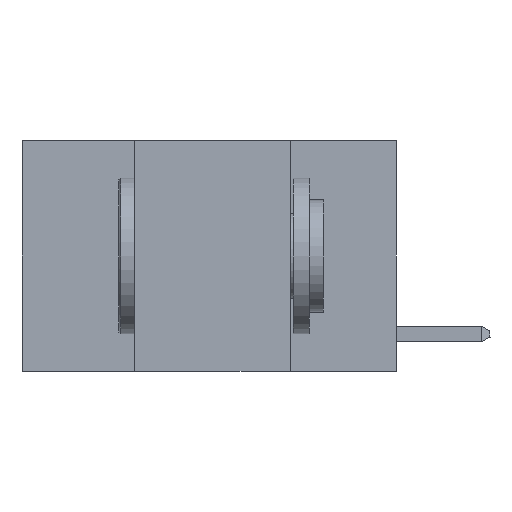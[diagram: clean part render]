
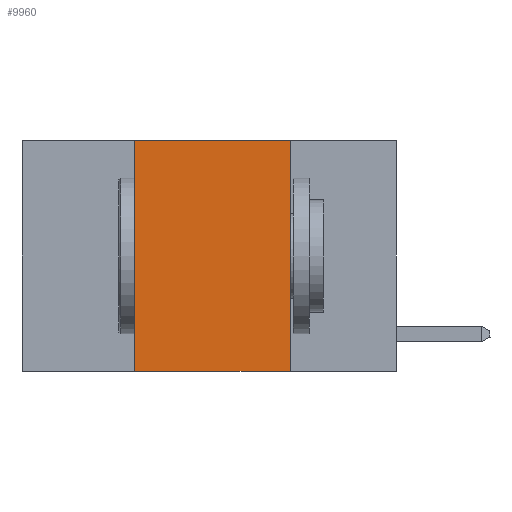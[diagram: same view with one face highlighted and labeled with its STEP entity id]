
A CAD part, left-side view. The second image highlights one B-rep face of the part: STEP entity #9960.
In plain terms, the highlighted planar face has unit normal (-1, 0, 0).
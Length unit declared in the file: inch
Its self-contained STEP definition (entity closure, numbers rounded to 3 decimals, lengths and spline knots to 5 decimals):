
#181 = DIRECTION ( 'NONE',  ( 0., 0., -1. ) ) ;
#400 = ORIENTED_EDGE ( 'NONE', *, *, #8873, .F. ) ;
#420 = LINE ( 'NONE', #10847, #8089 ) ;
#532 = DIRECTION ( 'NONE',  ( 0., -1., 0. ) ) ;
#733 = ORIENTED_EDGE ( 'NONE', *, *, #2205, .F. ) ;
#855 = LINE ( 'NONE', #8865, #3479 ) ;
#1025 = LINE ( 'NONE', #4388, #5730 ) ;
#1052 = DIRECTION ( 'NONE',  ( 1., 0., 0. ) ) ;
#1466 = ORIENTED_EDGE ( 'NONE', *, *, #10850, .F. ) ;
#2003 = VERTEX_POINT ( 'NONE', #9955 ) ;
#2205 = EDGE_CURVE ( 'NONE', #6620, #8295, #2412, .T. ) ;
#2412 = LINE ( 'NONE', #8538, #4542 ) ;
#3479 = VECTOR ( 'NONE', #5262, 39.37008 ) ;
#3792 = FACE_OUTER_BOUND ( 'NONE', #8815, .T. ) ;
#4388 = CARTESIAN_POINT ( 'NONE',  ( 0., 0.17, 0. ) ) ;
#4542 = VECTOR ( 'NONE', #532, 39.37008 ) ;
#5262 = DIRECTION ( 'NONE',  ( 0., -1., 0. ) ) ;
#5730 = VECTOR ( 'NONE', #7804, 39.37008 ) ;
#6620 = VERTEX_POINT ( 'NONE', #9179 ) ;
#7317 = ORIENTED_EDGE ( 'NONE', *, *, #7428, .T. ) ;
#7428 = EDGE_CURVE ( 'NONE', #2003, #10250, #855, .T. ) ;
#7804 = DIRECTION ( 'NONE',  ( 0., 0., -1. ) ) ;
#8089 = VECTOR ( 'NONE', #10003, 39.37008 ) ;
#8295 = VERTEX_POINT ( 'NONE', #10362 ) ;
#8538 = CARTESIAN_POINT ( 'NONE',  ( 0., 0.6, 0. ) ) ;
#8815 = EDGE_LOOP ( 'NONE', ( #400, #733, #1466, #7317 ) ) ;
#8865 = CARTESIAN_POINT ( 'NONE',  ( 0., 0.6, -0.37 ) ) ;
#8873 = EDGE_CURVE ( 'NONE', #8295, #10250, #1025, .T. ) ;
#9179 = CARTESIAN_POINT ( 'NONE',  ( 0., 0.42, 0. ) ) ;
#9765 = CARTESIAN_POINT ( 'NONE',  ( 0., 0.6, 0. ) ) ;
#9823 = PLANE ( 'NONE',  #10103 ) ;
#9851 = CARTESIAN_POINT ( 'NONE',  ( 0., 0.17, -0.37 ) ) ;
#9955 = CARTESIAN_POINT ( 'NONE',  ( 0., 0.42, -0.37 ) ) ;
#9960 = ADVANCED_FACE ( 'NONE', ( #3792 ), #9823, .F. ) ;
#10003 = DIRECTION ( 'NONE',  ( 0., 0., 1. ) ) ;
#10103 = AXIS2_PLACEMENT_3D ( 'NONE', #9765, #1052, #181 ) ;
#10250 = VERTEX_POINT ( 'NONE', #9851 ) ;
#10362 = CARTESIAN_POINT ( 'NONE',  ( 0., 0.17, 0. ) ) ;
#10847 = CARTESIAN_POINT ( 'NONE',  ( 0., 0.42, 0. ) ) ;
#10850 = EDGE_CURVE ( 'NONE', #2003, #6620, #420, .T. ) ;
